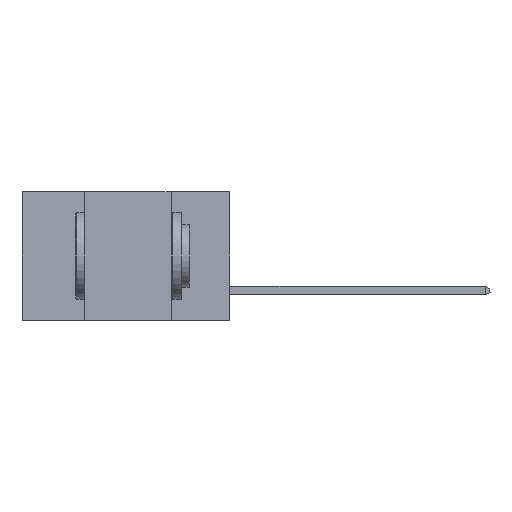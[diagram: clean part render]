
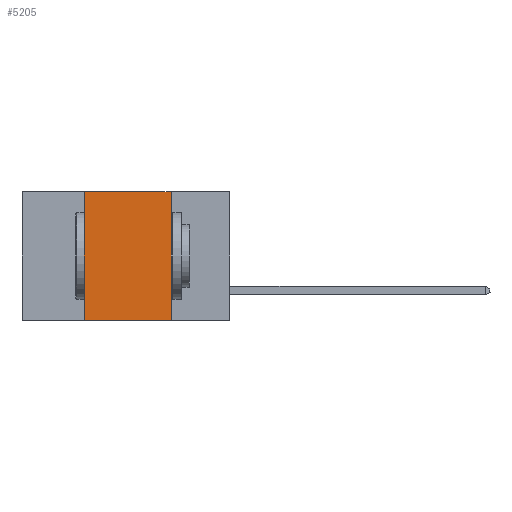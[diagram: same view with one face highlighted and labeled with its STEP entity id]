
A CAD part, left-side view. The second image highlights one B-rep face of the part: STEP entity #5205.
In plain terms, the highlighted planar face has unit normal (-1, 0, 0).
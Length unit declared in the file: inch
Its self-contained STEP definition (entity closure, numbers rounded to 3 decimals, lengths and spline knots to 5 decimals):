
#414 = EDGE_CURVE ( 'NONE', #9445, #5223, #7691, .T. ) ;
#1334 = VECTOR ( 'NONE', #14609, 39.37008 ) ;
#1758 = VECTOR ( 'NONE', #15001, 39.37008 ) ;
#1792 = ORIENTED_EDGE ( 'NONE', *, *, #8198, .F. ) ;
#2078 = CARTESIAN_POINT ( 'NONE',  ( 0., 0.17, 0. ) ) ;
#2516 = DIRECTION ( 'NONE',  ( 0., -1., 0. ) ) ;
#4335 = ORIENTED_EDGE ( 'NONE', *, *, #4499, .T. ) ;
#4499 = EDGE_CURVE ( 'NONE', #9445, #10992, #13741, .T. ) ;
#4923 = CARTESIAN_POINT ( 'NONE',  ( 0., 0.17, 0. ) ) ;
#5098 = EDGE_LOOP ( 'NONE', ( #1792, #13773, #5788, #4335 ) ) ;
#5174 = PLANE ( 'NONE',  #6932 ) ;
#5205 = ADVANCED_FACE ( 'NONE', ( #14684 ), #5174, .F. ) ;
#5223 = VERTEX_POINT ( 'NONE', #15068 ) ;
#5788 = ORIENTED_EDGE ( 'NONE', *, *, #414, .F. ) ;
#6071 = VECTOR ( 'NONE', #7599, 39.37008 ) ;
#6269 = DIRECTION ( 'NONE',  ( 1., 0., 0. ) ) ;
#6483 = CARTESIAN_POINT ( 'NONE',  ( 0., 0.6, 0. ) ) ;
#6932 = AXIS2_PLACEMENT_3D ( 'NONE', #6483, #6269, #14862 ) ;
#7599 = DIRECTION ( 'NONE',  ( 0., -1., 0. ) ) ;
#7691 = LINE ( 'NONE', #13552, #1758 ) ;
#7696 = CARTESIAN_POINT ( 'NONE',  ( 0., 0.6, 0. ) ) ;
#8198 = EDGE_CURVE ( 'NONE', #10828, #10992, #14352, .T. ) ;
#8443 = CARTESIAN_POINT ( 'NONE',  ( 0., 0.17, -0.37 ) ) ;
#9445 = VERTEX_POINT ( 'NONE', #11562 ) ;
#10828 = VERTEX_POINT ( 'NONE', #2078 ) ;
#10852 = VECTOR ( 'NONE', #2516, 39.37008 ) ;
#10992 = VERTEX_POINT ( 'NONE', #8443 ) ;
#11562 = CARTESIAN_POINT ( 'NONE',  ( 0., 0.42, -0.37 ) ) ;
#13315 = EDGE_CURVE ( 'NONE', #5223, #10828, #13758, .T. ) ;
#13552 = CARTESIAN_POINT ( 'NONE',  ( 0., 0.42, 0. ) ) ;
#13741 = LINE ( 'NONE', #14786, #10852 ) ;
#13758 = LINE ( 'NONE', #7696, #6071 ) ;
#13773 = ORIENTED_EDGE ( 'NONE', *, *, #13315, .F. ) ;
#14352 = LINE ( 'NONE', #4923, #1334 ) ;
#14609 = DIRECTION ( 'NONE',  ( 0., 0., -1. ) ) ;
#14684 = FACE_OUTER_BOUND ( 'NONE', #5098, .T. ) ;
#14786 = CARTESIAN_POINT ( 'NONE',  ( 0., 0.6, -0.37 ) ) ;
#14862 = DIRECTION ( 'NONE',  ( 0., 0., -1. ) ) ;
#15001 = DIRECTION ( 'NONE',  ( 0., 0., 1. ) ) ;
#15068 = CARTESIAN_POINT ( 'NONE',  ( 0., 0.42, 0. ) ) ;
